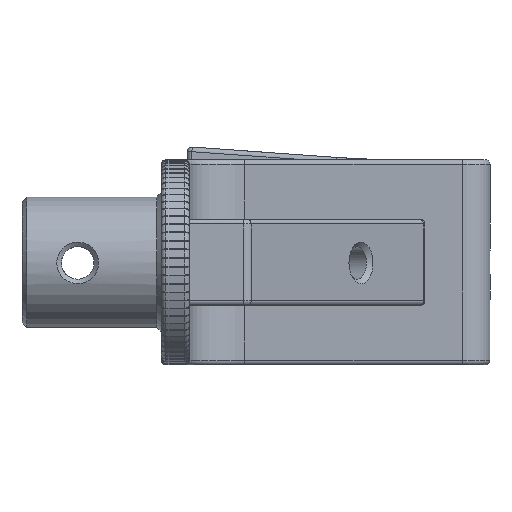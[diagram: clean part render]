
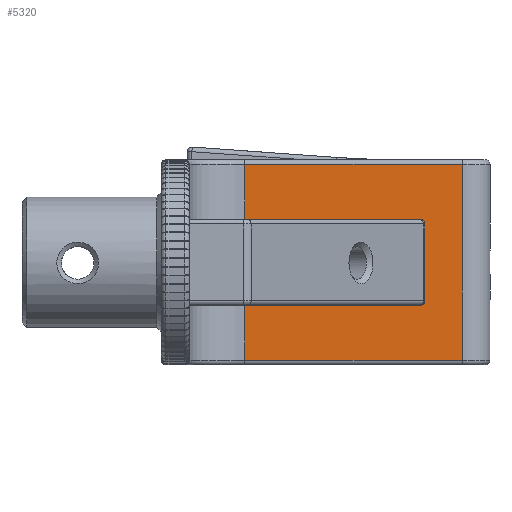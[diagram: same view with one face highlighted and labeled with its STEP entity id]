
A CAD part, left-side view. The second image highlights one B-rep face of the part: STEP entity #5320.
In plain terms, the highlighted planar face has unit normal (-1, 0, 0).
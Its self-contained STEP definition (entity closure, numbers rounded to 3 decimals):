
#191=PLANE('',#6004);
#719=FACE_OUTER_BOUND('',#1062,.T.);
#1062=EDGE_LOOP('',(#4962,#4963,#4964,#4965,#4966,#4967,#4968,#4969,#4970,
#4971));
#1114=LINE('',#7973,#1450);
#1123=LINE('',#8031,#1459);
#1125=LINE('',#8034,#1461);
#1344=LINE('',#10104,#1680);
#1384=LINE('',#10728,#1720);
#1398=LINE('',#10903,#1734);
#1399=LINE('',#10907,#1735);
#1400=LINE('',#10908,#1736);
#1450=VECTOR('',#6174,10.);
#1459=VECTOR('',#6215,10.);
#1461=VECTOR('',#6219,10.);
#1680=VECTOR('',#7242,10.);
#1720=VECTOR('',#7606,10.);
#1734=VECTOR('',#7672,10.);
#1735=VECTOR('',#7679,10.);
#1736=VECTOR('',#7680,10.);
#1779=CIRCLE('',#5383,0.5);
#1798=CIRCLE('',#5408,0.5);
#2248=VERTEX_POINT('',#7926);
#2249=VERTEX_POINT('',#7928);
#2258=VERTEX_POINT('',#7972);
#2270=VERTEX_POINT('',#8021);
#2271=VERTEX_POINT('',#8022);
#2273=VERTEX_POINT('',#8029);
#2524=VERTEX_POINT('',#10098);
#2525=VERTEX_POINT('',#10102);
#2604=VERTEX_POINT('',#10722);
#2605=VERTEX_POINT('',#10726);
#2703=EDGE_CURVE('',#2248,#2249,#1779,.F.);
#2717=EDGE_CURVE('',#2258,#2249,#1114,.T.);
#2733=EDGE_CURVE('',#2270,#2271,#1798,.F.);
#2738=EDGE_CURVE('',#2270,#2273,#1123,.T.);
#2740=EDGE_CURVE('',#2271,#2248,#1125,.T.);
#3213=EDGE_CURVE('',#2524,#2525,#1344,.T.);
#3373=EDGE_CURVE('',#2604,#2605,#1384,.T.);
#3399=EDGE_CURVE('',#2605,#2524,#1398,.T.);
#3400=EDGE_CURVE('',#2258,#2604,#1399,.T.);
#3401=EDGE_CURVE('',#2525,#2273,#1400,.T.);
#4962=ORIENTED_EDGE('',*,*,#3213,.F.);
#4963=ORIENTED_EDGE('',*,*,#3399,.F.);
#4964=ORIENTED_EDGE('',*,*,#3373,.F.);
#4965=ORIENTED_EDGE('',*,*,#3400,.F.);
#4966=ORIENTED_EDGE('',*,*,#2717,.T.);
#4967=ORIENTED_EDGE('',*,*,#2703,.F.);
#4968=ORIENTED_EDGE('',*,*,#2740,.F.);
#4969=ORIENTED_EDGE('',*,*,#2733,.F.);
#4970=ORIENTED_EDGE('',*,*,#2738,.T.);
#4971=ORIENTED_EDGE('',*,*,#3401,.F.);
#5320=ADVANCED_FACE('',(#719),#191,.F.);
#5383=AXIS2_PLACEMENT_3D('',#7929,#6145,#6146);
#5408=AXIS2_PLACEMENT_3D('',#8023,#6206,#6207);
#6004=AXIS2_PLACEMENT_3D('',#10906,#7677,#7678);
#6145=DIRECTION('center_axis',(1.,0.,0.));
#6146=DIRECTION('ref_axis',(0.,-0.707,0.707));
#6174=DIRECTION('',(0.,-1.,0.));
#6206=DIRECTION('center_axis',(1.,0.,0.));
#6207=DIRECTION('ref_axis',(0.,-0.707,-0.707));
#6215=DIRECTION('',(0.,1.,0.));
#6219=DIRECTION('',(0.,0.,1.));
#7242=DIRECTION('',(0.,1.,0.));
#7606=DIRECTION('',(0.,-1.,0.));
#7672=DIRECTION('',(0.,0.,-1.));
#7677=DIRECTION('center_axis',(1.,0.,0.));
#7678=DIRECTION('ref_axis',(0.,0.,-1.));
#7679=DIRECTION('',(0.,0.,1.));
#7680=DIRECTION('',(0.,0.,1.));
#7926=CARTESIAN_POINT('',(87.258,-27.46,46.885));
#7928=CARTESIAN_POINT('',(87.258,-26.96,47.385));
#7929=CARTESIAN_POINT('Origin',(87.258,-26.96,46.885));
#7972=CARTESIAN_POINT('',(87.258,-8.06,47.385));
#7973=CARTESIAN_POINT('',(87.258,-20.66,47.385));
#8021=CARTESIAN_POINT('',(87.258,-26.96,38.115));
#8022=CARTESIAN_POINT('',(87.258,-27.46,38.615));
#8023=CARTESIAN_POINT('Origin',(87.258,-26.96,38.615));
#8029=CARTESIAN_POINT('',(87.258,-8.06,38.115));
#8031=CARTESIAN_POINT('',(87.258,-20.66,38.115));
#8034=CARTESIAN_POINT('',(87.258,-27.46,53.799));
#10098=CARTESIAN_POINT('',(87.258,-31.46,32.201));
#10102=CARTESIAN_POINT('',(87.258,-8.06,32.201));
#10104=CARTESIAN_POINT('',(87.258,-20.36,32.201));
#10722=CARTESIAN_POINT('',(87.258,-8.06,53.299));
#10726=CARTESIAN_POINT('',(87.258,-31.46,53.299));
#10728=CARTESIAN_POINT('',(87.258,-7.66,53.299));
#10903=CARTESIAN_POINT('',(87.258,-31.46,42.75));
#10906=CARTESIAN_POINT('Origin',(87.258,-13.26,42.75));
#10907=CARTESIAN_POINT('',(87.258,-8.06,45.125));
#10908=CARTESIAN_POINT('',(87.258,-8.06,45.125));
